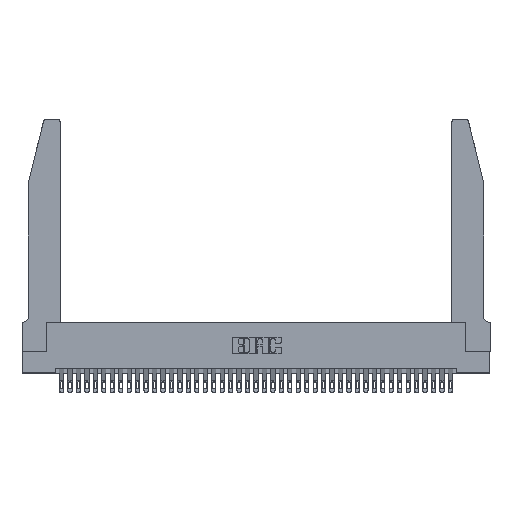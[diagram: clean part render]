
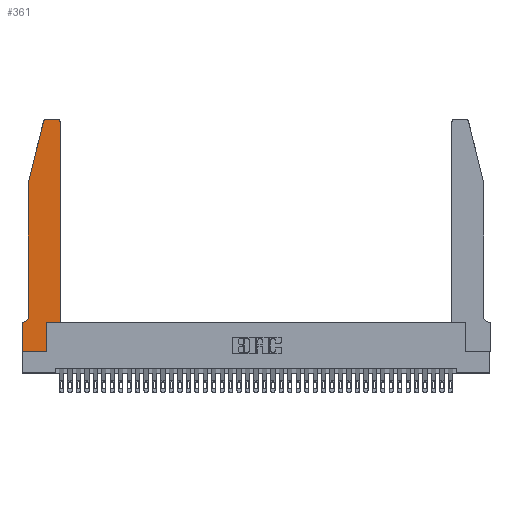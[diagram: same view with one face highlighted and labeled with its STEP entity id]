
A CAD part, top view. The second image highlights one B-rep face of the part: STEP entity #361.
In plain terms, the highlighted planar face has unit normal (0, 0, 1).
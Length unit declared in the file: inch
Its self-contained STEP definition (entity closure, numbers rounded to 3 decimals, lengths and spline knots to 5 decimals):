
#165 = VERTEX_POINT ( 'NONE', #21659 ) ;
#260 = DIRECTION ( 'NONE',  ( -0.239, -0.971, 0. ) ) ;
#361 = ADVANCED_FACE ( 'NONE', ( #39095 ), #26272, .T. ) ;
#1191 = VERTEX_POINT ( 'NONE', #36247 ) ;
#1284 = EDGE_CURVE ( 'NONE', #6708, #11022, #26385, .T. ) ;
#1296 = ORIENTED_EDGE ( 'NONE', *, *, #2727, .T. ) ;
#1864 = CARTESIAN_POINT ( 'NONE',  ( 0.4505, 2.72, 0.37 ) ) ;
#2597 = LINE ( 'NONE', #5319, #12369 ) ;
#2727 = EDGE_CURVE ( 'NONE', #33174, #6708, #2597, .T. ) ;
#3019 = CARTESIAN_POINT ( 'NONE',  ( 0.284, 2.72, 0.37 ) ) ;
#3544 = ORIENTED_EDGE ( 'NONE', *, *, #14056, .T. ) ;
#3707 = CARTESIAN_POINT ( 'NONE',  ( 0.2865, 0., 0.37 ) ) ;
#3757 = EDGE_CURVE ( 'NONE', #14856, #33174, #27618, .T. ) ;
#4261 = CARTESIAN_POINT ( 'NONE',  ( 0.2865, 0.35, 0.37 ) ) ;
#5319 = CARTESIAN_POINT ( 'NONE',  ( 0.4505, 0.35, 0.37 ) ) ;
#6345 = DIRECTION ( 'NONE',  ( 1., 0., 0. ) ) ;
#6708 = VERTEX_POINT ( 'NONE', #1864 ) ;
#7334 = LINE ( 'NONE', #35957, #31727 ) ;
#8427 = DIRECTION ( 'NONE',  ( 0., 0., 1. ) ) ;
#11010 = EDGE_CURVE ( 'NONE', #35123, #27331, #17463, .T. ) ;
#11022 = VERTEX_POINT ( 'NONE', #29616 ) ;
#11423 = CARTESIAN_POINT ( 'NONE',  ( 0., 0., 0.37 ) ) ;
#11988 = VECTOR ( 'NONE', #39326, 39.37008 ) ;
#12014 = EDGE_LOOP ( 'NONE', ( #38628, #3544, #32434, #34838, #27676, #13598, #33170, #31596, #30002, #27151, #1296, #26956 ) ) ;
#12369 = VECTOR ( 'NONE', #24561, 39.37008 ) ;
#12692 = DIRECTION ( 'NONE',  ( 1., 0., 0. ) ) ;
#13075 = VECTOR ( 'NONE', #31957, 39.37008 ) ;
#13209 = CARTESIAN_POINT ( 'NONE',  ( 0.0055, 0.42, 0.37 ) ) ;
#13284 = AXIS2_PLACEMENT_3D ( 'NONE', #27548, #8427, #30674 ) ;
#13598 = ORIENTED_EDGE ( 'NONE', *, *, #34613, .T. ) ;
#14056 = EDGE_CURVE ( 'NONE', #19222, #165, #24582, .T. ) ;
#14079 = CARTESIAN_POINT ( 'NONE',  ( 0., 0.35, 0.37 ) ) ;
#14828 = DIRECTION ( 'NONE',  ( -1., 0., 0. ) ) ;
#14856 = VERTEX_POINT ( 'NONE', #4261 ) ;
#15377 = CARTESIAN_POINT ( 'NONE',  ( 0.0755, 2., 0.37 ) ) ;
#16201 = CARTESIAN_POINT ( 'NONE',  ( 0., 0., 0.37 ) ) ;
#16457 = DIRECTION ( 'NONE',  ( -1., 0., 0. ) ) ;
#16507 = VECTOR ( 'NONE', #14828, 39.37008 ) ;
#16705 = VECTOR ( 'NONE', #19372, 39.37008 ) ;
#16974 = DIRECTION ( 'NONE',  ( 0., -1., 0. ) ) ;
#17187 = AXIS2_PLACEMENT_3D ( 'NONE', #3019, #25540, #6345 ) ;
#17463 = LINE ( 'NONE', #20154, #33138 ) ;
#18674 = EDGE_CURVE ( 'NONE', #27331, #26737, #33388, .T. ) ;
#19222 = VERTEX_POINT ( 'NONE', #38588 ) ;
#19242 = VECTOR ( 'NONE', #38295, 39.37008 ) ;
#19372 = DIRECTION ( 'NONE',  ( 1., 0., 0. ) ) ;
#20154 = CARTESIAN_POINT ( 'NONE',  ( 0., 0., 0.37 ) ) ;
#20479 = LINE ( 'NONE', #26846, #11988 ) ;
#21513 = AXIS2_PLACEMENT_3D ( 'NONE', #14079, #22073, #12692 ) ;
#21588 = EDGE_CURVE ( 'NONE', #1191, #38466, #28286, .T. ) ;
#21659 = CARTESIAN_POINT ( 'NONE',  ( 0.25487, 2.72718, 0.37 ) ) ;
#21840 = LINE ( 'NONE', #38487, #37445 ) ;
#22073 = DIRECTION ( 'NONE',  ( 0., 0., 1. ) ) ;
#23090 = CARTESIAN_POINT ( 'NONE',  ( 0.4505, 0.35, 0.37 ) ) ;
#24561 = DIRECTION ( 'NONE',  ( 0., 1., 0. ) ) ;
#24582 = CIRCLE ( 'NONE', #17187, 0.03 ) ;
#25540 = DIRECTION ( 'NONE',  ( 0., 0., 1. ) ) ;
#26272 = PLANE ( 'NONE',  #21513 ) ;
#26382 = CARTESIAN_POINT ( 'NONE',  ( 0., 0.35, 0.37 ) ) ;
#26385 = CIRCLE ( 'NONE', #13284, 0.03 ) ;
#26737 = VERTEX_POINT ( 'NONE', #3707 ) ;
#26846 = CARTESIAN_POINT ( 'NONE',  ( 0.0755, 0.35, 0.37 ) ) ;
#26956 = ORIENTED_EDGE ( 'NONE', *, *, #1284, .T. ) ;
#27151 = ORIENTED_EDGE ( 'NONE', *, *, #3757, .T. ) ;
#27328 = CARTESIAN_POINT ( 'NONE',  ( 0.0055, 0.35, 0.37 ) ) ;
#27331 = VERTEX_POINT ( 'NONE', #11423 ) ;
#27548 = CARTESIAN_POINT ( 'NONE',  ( 0.4205, 2.72, 0.37 ) ) ;
#27604 = EDGE_CURVE ( 'NONE', #26737, #14856, #30873, .T. ) ;
#27618 = LINE ( 'NONE', #32052, #19242 ) ;
#27676 = ORIENTED_EDGE ( 'NONE', *, *, #21588, .T. ) ;
#28286 = CIRCLE ( 'NONE', #41235, 0.07 ) ;
#29436 = EDGE_CURVE ( 'NONE', #165, #39523, #21840, .T. ) ;
#29616 = CARTESIAN_POINT ( 'NONE',  ( 0.4205, 2.75, 0.37 ) ) ;
#30002 = ORIENTED_EDGE ( 'NONE', *, *, #27604, .T. ) ;
#30674 = DIRECTION ( 'NONE',  ( 1., 0., 0. ) ) ;
#30873 = LINE ( 'NONE', #35207, #13075 ) ;
#31596 = ORIENTED_EDGE ( 'NONE', *, *, #18674, .T. ) ;
#31727 = VECTOR ( 'NONE', #32836, 39.37008 ) ;
#31957 = DIRECTION ( 'NONE',  ( 0., 1., 0. ) ) ;
#32052 = CARTESIAN_POINT ( 'NONE',  ( 0.4505, 0.35, 0.37 ) ) ;
#32434 = ORIENTED_EDGE ( 'NONE', *, *, #29436, .T. ) ;
#32836 = DIRECTION ( 'NONE',  ( 0., -1., 0. ) ) ;
#33138 = VECTOR ( 'NONE', #16974, 39.37008 ) ;
#33170 = ORIENTED_EDGE ( 'NONE', *, *, #11010, .T. ) ;
#33174 = VERTEX_POINT ( 'NONE', #23090 ) ;
#33195 = LINE ( 'NONE', #33619, #16507 ) ;
#33388 = LINE ( 'NONE', #16201, #16705 ) ;
#33619 = CARTESIAN_POINT ( 'NONE',  ( 0.2605, 2.75, 0.37 ) ) ;
#34613 = EDGE_CURVE ( 'NONE', #38466, #35123, #20479, .T. ) ;
#34722 = EDGE_CURVE ( 'NONE', #11022, #19222, #33195, .T. ) ;
#34838 = ORIENTED_EDGE ( 'NONE', *, *, #37096, .T. ) ;
#35123 = VERTEX_POINT ( 'NONE', #26382 ) ;
#35207 = CARTESIAN_POINT ( 'NONE',  ( 0.2865, 0.35, 0.37 ) ) ;
#35209 = DIRECTION ( 'NONE',  ( 0., 0., -1. ) ) ;
#35957 = CARTESIAN_POINT ( 'NONE',  ( 0.0755, 2., 0.37 ) ) ;
#36247 = CARTESIAN_POINT ( 'NONE',  ( 0.0755, 0.42, 0.37 ) ) ;
#37096 = EDGE_CURVE ( 'NONE', #39523, #1191, #7334, .T. ) ;
#37445 = VECTOR ( 'NONE', #260, 39.37008 ) ;
#38295 = DIRECTION ( 'NONE',  ( 1., 0., 0. ) ) ;
#38466 = VERTEX_POINT ( 'NONE', #27328 ) ;
#38487 = CARTESIAN_POINT ( 'NONE',  ( 0.0755, 2., 0.37 ) ) ;
#38588 = CARTESIAN_POINT ( 'NONE',  ( 0.284, 2.75, 0.37 ) ) ;
#38628 = ORIENTED_EDGE ( 'NONE', *, *, #34722, .T. ) ;
#39095 = FACE_OUTER_BOUND ( 'NONE', #12014, .T. ) ;
#39326 = DIRECTION ( 'NONE',  ( -1., 0., 0. ) ) ;
#39523 = VERTEX_POINT ( 'NONE', #15377 ) ;
#41235 = AXIS2_PLACEMENT_3D ( 'NONE', #13209, #35209, #16457 ) ;
